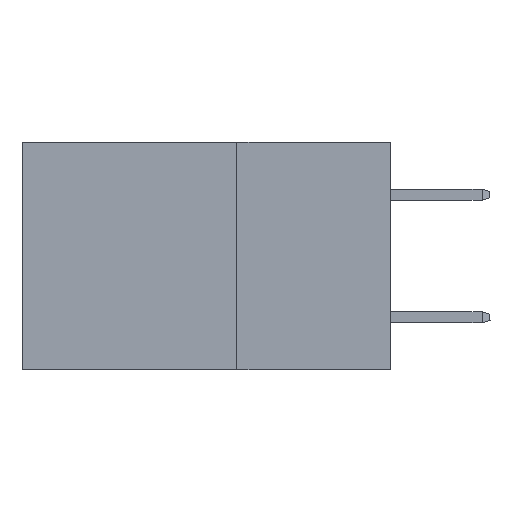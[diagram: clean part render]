
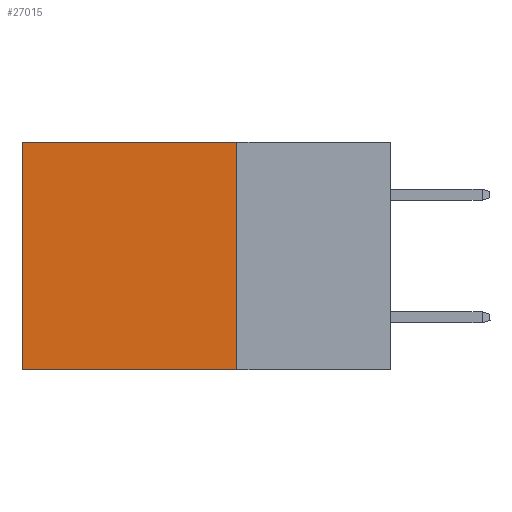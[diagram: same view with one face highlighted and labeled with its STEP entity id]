
A CAD part, left-side view. The second image highlights one B-rep face of the part: STEP entity #27015.
In plain terms, the highlighted planar face has unit normal (-1, 0, 0).
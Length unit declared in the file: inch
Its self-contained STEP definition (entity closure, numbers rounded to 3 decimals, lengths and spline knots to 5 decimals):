
#1098 = CARTESIAN_POINT ( 'NONE',  ( 0.2875, 0.25, 0. ) ) ;
#1524 = ORIENTED_EDGE ( 'NONE', *, *, #2349, .T. ) ;
#2349 = EDGE_CURVE ( 'NONE', #39683, #35208, #39018, .T. ) ;
#2850 = ORIENTED_EDGE ( 'NONE', *, *, #25797, .T. ) ;
#3749 = EDGE_LOOP ( 'NONE', ( #1524, #35795, #29402, #2850 ) ) ;
#4342 = VECTOR ( 'NONE', #18608, 39.37008 ) ;
#4596 = LINE ( 'NONE', #32262, #23730 ) ;
#5537 = CARTESIAN_POINT ( 'NONE',  ( 0.2875, 0.25, -0.37 ) ) ;
#6129 = DIRECTION ( 'NONE',  ( 0., 1., 0. ) ) ;
#6924 = DIRECTION ( 'NONE',  ( 0., 0., -1. ) ) ;
#9373 = AXIS2_PLACEMENT_3D ( 'NONE', #26702, #26276, #6924 ) ;
#10574 = CARTESIAN_POINT ( 'NONE',  ( 0.2875, 0.25, 0. ) ) ;
#11135 = CARTESIAN_POINT ( 'NONE',  ( 0.2875, 0.6, 0. ) ) ;
#11669 = VERTEX_POINT ( 'NONE', #10574 ) ;
#14240 = VERTEX_POINT ( 'NONE', #5537 ) ;
#15440 = CARTESIAN_POINT ( 'NONE',  ( 0.2875, 0.6, 0. ) ) ;
#18608 = DIRECTION ( 'NONE',  ( 0., 0., -1. ) ) ;
#18841 = EDGE_CURVE ( 'NONE', #11669, #14240, #31485, .T. ) ;
#20751 = DIRECTION ( 'NONE',  ( 0., 0., -1. ) ) ;
#21035 = DIRECTION ( 'NONE',  ( 0., 1., 0. ) ) ;
#22022 = CARTESIAN_POINT ( 'NONE',  ( 0.2875, 0.6, -0.37 ) ) ;
#23412 = PLANE ( 'NONE',  #9373 ) ;
#23730 = VECTOR ( 'NONE', #6129, 39.37008 ) ;
#25797 = EDGE_CURVE ( 'NONE', #11669, #39683, #30269, .T. ) ;
#26276 = DIRECTION ( 'NONE',  ( 1., 0., 0. ) ) ;
#26702 = CARTESIAN_POINT ( 'NONE',  ( 0.2875, 0.25, 0. ) ) ;
#27015 = ADVANCED_FACE ( 'NONE', ( #34416 ), #23412, .F. ) ;
#29402 = ORIENTED_EDGE ( 'NONE', *, *, #18841, .F. ) ;
#29946 = VECTOR ( 'NONE', #20751, 39.37008 ) ;
#30269 = LINE ( 'NONE', #1098, #38559 ) ;
#31485 = LINE ( 'NONE', #40564, #29946 ) ;
#32262 = CARTESIAN_POINT ( 'NONE',  ( 0.2875, 0.25, -0.37 ) ) ;
#34416 = FACE_OUTER_BOUND ( 'NONE', #3749, .T. ) ;
#35208 = VERTEX_POINT ( 'NONE', #22022 ) ;
#35795 = ORIENTED_EDGE ( 'NONE', *, *, #36674, .F. ) ;
#36674 = EDGE_CURVE ( 'NONE', #14240, #35208, #4596, .T. ) ;
#38559 = VECTOR ( 'NONE', #21035, 39.37008 ) ;
#39018 = LINE ( 'NONE', #15440, #4342 ) ;
#39683 = VERTEX_POINT ( 'NONE', #11135 ) ;
#40564 = CARTESIAN_POINT ( 'NONE',  ( 0.2875, 0.25, 0. ) ) ;
